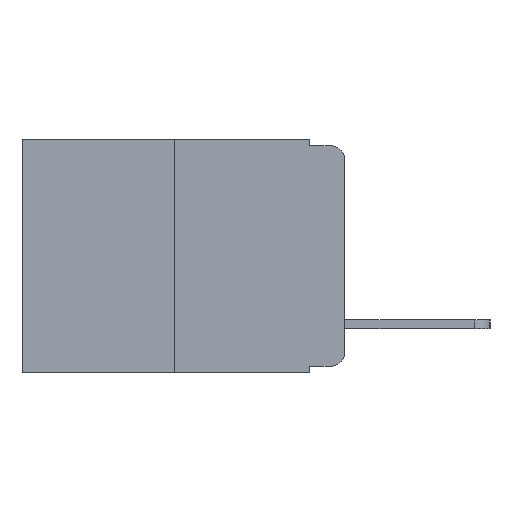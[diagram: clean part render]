
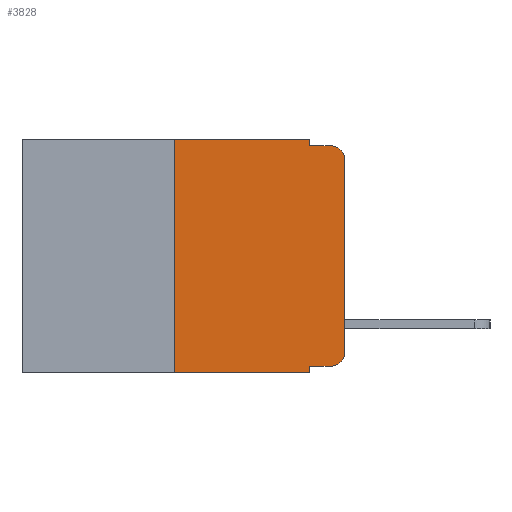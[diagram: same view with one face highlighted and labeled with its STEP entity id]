
A CAD part, left-side view. The second image highlights one B-rep face of the part: STEP entity #3828.
In plain terms, the highlighted planar face has unit normal (-1, 0, 0).
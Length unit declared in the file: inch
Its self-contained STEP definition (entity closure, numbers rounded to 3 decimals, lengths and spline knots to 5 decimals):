
#9 = EDGE_CURVE ( 'NONE', #11438, #8084, #2794, .T. ) ;
#317 = DIRECTION ( 'NONE',  ( 0., 0., -1. ) ) ;
#359 = VERTEX_POINT ( 'NONE', #10380 ) ;
#396 = EDGE_CURVE ( 'NONE', #5935, #2975, #4560, .T. ) ;
#549 = DIRECTION ( 'NONE',  ( 0., -1., 0. ) ) ;
#597 = EDGE_CURVE ( 'NONE', #2814, #2975, #3233, .T. ) ;
#1066 = ORIENTED_EDGE ( 'NONE', *, *, #3425, .T. ) ;
#1125 = VECTOR ( 'NONE', #8659, 39.37008 ) ;
#1160 = EDGE_CURVE ( 'NONE', #1438, #2681, #3051, .T. ) ;
#1340 = ORIENTED_EDGE ( 'NONE', *, *, #4455, .T. ) ;
#1352 = LINE ( 'NONE', #6047, #3427 ) ;
#1438 = VERTEX_POINT ( 'NONE', #9822 ) ;
#1879 = CARTESIAN_POINT ( 'NONE',  ( 0., 0.051, 0. ) ) ;
#2046 = ORIENTED_EDGE ( 'NONE', *, *, #8243, .F. ) ;
#2113 = VECTOR ( 'NONE', #7494, 39.37008 ) ;
#2236 = CARTESIAN_POINT ( 'NONE',  ( 0., 0.473, 0. ) ) ;
#2250 = CARTESIAN_POINT ( 'NONE',  ( 0., 0., 0. ) ) ;
#2288 = VECTOR ( 'NONE', #3800, 39.37008 ) ;
#2681 = VERTEX_POINT ( 'NONE', #4735 ) ;
#2794 = LINE ( 'NONE', #2250, #7413 ) ;
#2805 = AXIS2_PLACEMENT_3D ( 'NONE', #8566, #3200, #9377 ) ;
#2814 = VERTEX_POINT ( 'NONE', #11710 ) ;
#2841 = CARTESIAN_POINT ( 'NONE',  ( 0., 0.02, -0.01 ) ) ;
#2975 = VERTEX_POINT ( 'NONE', #7256 ) ;
#3051 = LINE ( 'NONE', #5116, #9782 ) ;
#3200 = DIRECTION ( 'NONE',  ( -1., 0., 0. ) ) ;
#3208 = CARTESIAN_POINT ( 'NONE',  ( 0., 0.473, -0.343 ) ) ;
#3233 = LINE ( 'NONE', #11753, #11551 ) ;
#3259 = DIRECTION ( 'NONE',  ( 1., 0., 0. ) ) ;
#3425 = EDGE_CURVE ( 'NONE', #359, #11438, #4234, .T. ) ;
#3427 = VECTOR ( 'NONE', #5147, 39.37008 ) ;
#3757 = ORIENTED_EDGE ( 'NONE', *, *, #396, .T. ) ;
#3800 = DIRECTION ( 'NONE',  ( 0., -1., 0. ) ) ;
#3828 = ADVANCED_FACE ( 'NONE', ( #7210 ), #7805, .F. ) ;
#4234 = CIRCLE ( 'NONE', #11009, 0.02 ) ;
#4455 = EDGE_CURVE ( 'NONE', #8084, #7743, #9752, .T. ) ;
#4560 = LINE ( 'NONE', #3208, #2288 ) ;
#4735 = CARTESIAN_POINT ( 'NONE',  ( 0., 0.051, 0. ) ) ;
#5116 = CARTESIAN_POINT ( 'NONE',  ( 0., 0.473, 0. ) ) ;
#5147 = DIRECTION ( 'NONE',  ( 0., -1., 0. ) ) ;
#5443 = ORIENTED_EDGE ( 'NONE', *, *, #9, .T. ) ;
#5807 = ORIENTED_EDGE ( 'NONE', *, *, #8793, .F. ) ;
#5935 = VERTEX_POINT ( 'NONE', #6621 ) ;
#6047 = CARTESIAN_POINT ( 'NONE',  ( 0., 0.051, -0.01 ) ) ;
#6194 = DIRECTION ( 'NONE',  ( 0., 0., -1. ) ) ;
#6291 = DIRECTION ( 'NONE',  ( -1., 0., 0. ) ) ;
#6422 = DIRECTION ( 'NONE',  ( 0., -1., 0. ) ) ;
#6573 = ORIENTED_EDGE ( 'NONE', *, *, #597, .F. ) ;
#6621 = CARTESIAN_POINT ( 'NONE',  ( 0., 0.25, -0.343 ) ) ;
#6748 = VECTOR ( 'NONE', #549, 39.37008 ) ;
#7210 = FACE_OUTER_BOUND ( 'NONE', #10051, .T. ) ;
#7256 = CARTESIAN_POINT ( 'NONE',  ( 0., 0.051, -0.343 ) ) ;
#7361 = ORIENTED_EDGE ( 'NONE', *, *, #11662, .T. ) ;
#7393 = LINE ( 'NONE', #1879, #2113 ) ;
#7413 = VECTOR ( 'NONE', #10217, 39.37008 ) ;
#7494 = DIRECTION ( 'NONE',  ( 0., 0., -1. ) ) ;
#7688 = CARTESIAN_POINT ( 'NONE',  ( 0., 0.051, -0.01 ) ) ;
#7743 = VERTEX_POINT ( 'NONE', #2841 ) ;
#7805 = PLANE ( 'NONE',  #10801 ) ;
#7854 = CARTESIAN_POINT ( 'NONE',  ( 0., 0.25, 0. ) ) ;
#8084 = VERTEX_POINT ( 'NONE', #10080 ) ;
#8205 = LINE ( 'NONE', #11359, #6748 ) ;
#8243 = EDGE_CURVE ( 'NONE', #5935, #1438, #10676, .T. ) ;
#8566 = CARTESIAN_POINT ( 'NONE',  ( 0., 0.02, -0.03 ) ) ;
#8659 = DIRECTION ( 'NONE',  ( 0., 0., 1. ) ) ;
#8793 = EDGE_CURVE ( 'NONE', #2681, #11090, #7393, .T. ) ;
#9377 = DIRECTION ( 'NONE',  ( 0., 0., -1. ) ) ;
#9425 = DIRECTION ( 'NONE',  ( 0., 0., -1. ) ) ;
#9568 = CARTESIAN_POINT ( 'NONE',  ( 0., 0., -0.313 ) ) ;
#9752 = CIRCLE ( 'NONE', #2805, 0.02 ) ;
#9782 = VECTOR ( 'NONE', #6422, 39.37008 ) ;
#9822 = CARTESIAN_POINT ( 'NONE',  ( 0., 0.25, 0. ) ) ;
#10051 = EDGE_LOOP ( 'NONE', ( #5443, #1340, #10949, #5807, #11175, #2046, #3757, #6573, #7361, #1066 ) ) ;
#10080 = CARTESIAN_POINT ( 'NONE',  ( 0., 0., -0.03 ) ) ;
#10217 = DIRECTION ( 'NONE',  ( 0., 0., 1. ) ) ;
#10380 = CARTESIAN_POINT ( 'NONE',  ( 0., 0.02, -0.333 ) ) ;
#10676 = LINE ( 'NONE', #7854, #1125 ) ;
#10801 = AXIS2_PLACEMENT_3D ( 'NONE', #2236, #3259, #9425 ) ;
#10909 = EDGE_CURVE ( 'NONE', #11090, #7743, #1352, .T. ) ;
#10949 = ORIENTED_EDGE ( 'NONE', *, *, #10909, .F. ) ;
#11009 = AXIS2_PLACEMENT_3D ( 'NONE', #11201, #6291, #317 ) ;
#11090 = VERTEX_POINT ( 'NONE', #7688 ) ;
#11175 = ORIENTED_EDGE ( 'NONE', *, *, #1160, .F. ) ;
#11201 = CARTESIAN_POINT ( 'NONE',  ( 0., 0.02, -0.313 ) ) ;
#11359 = CARTESIAN_POINT ( 'NONE',  ( 0., 0.051, -0.333 ) ) ;
#11438 = VERTEX_POINT ( 'NONE', #9568 ) ;
#11551 = VECTOR ( 'NONE', #6194, 39.37008 ) ;
#11662 = EDGE_CURVE ( 'NONE', #2814, #359, #8205, .T. ) ;
#11710 = CARTESIAN_POINT ( 'NONE',  ( 0., 0.051, -0.333 ) ) ;
#11753 = CARTESIAN_POINT ( 'NONE',  ( 0., 0.051, 0. ) ) ;
